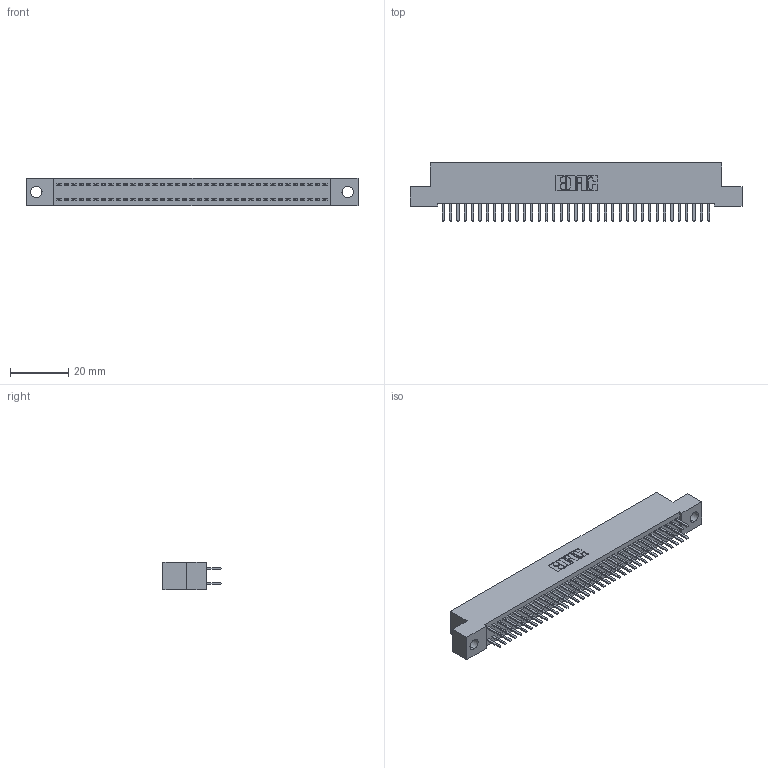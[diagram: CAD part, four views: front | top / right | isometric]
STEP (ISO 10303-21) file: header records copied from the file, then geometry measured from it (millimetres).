
FILE_DESCRIPTION (( 'STEP AP203' ), '1' );
FILE_NAME ('392-074-520-204.STEP', '2018-08-18T00:32:06', ( '' ), ( '' ), 'SwSTEP 2.0', 'SolidWorks 2016', '' );
FILE_SCHEMA (( 'CONFIG_CONTROL_DESIGN' ));
Length unit declared in the file: inch
Products named in the file (3): 342 Part_.156 TH; 345-292-001_345-293-120; 392-074-520-204
Assembly tree (75 placements, depth 2):
  392-074-520-204
    342 Part_.156 TH
    345-292-001_345-293-120  x74
Bounding box: 114.3 x 20.02 x 9.4 mm (x, y, z)
Volume: 10126.6 mm3; surface area: 16107.8 mm2
Topology: 75 solids, 75 shells, 4254 faces, 12361 edges, 8042 vertices
Faces by surface type: plane 2878, cylinder 1376
Entity records: 24435 total; most frequent: CARTESIAN_POINT 4066, ORIENTED_EDGE 3990, DIRECTION 3471, EDGE_CURVE 1995, VECTOR 1863, LINE 1863, VERTEX_POINT 1326, AXIS2_PLACEMENT_3D 804
